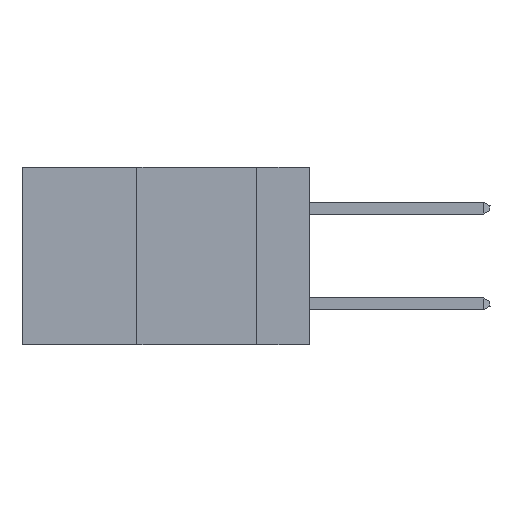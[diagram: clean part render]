
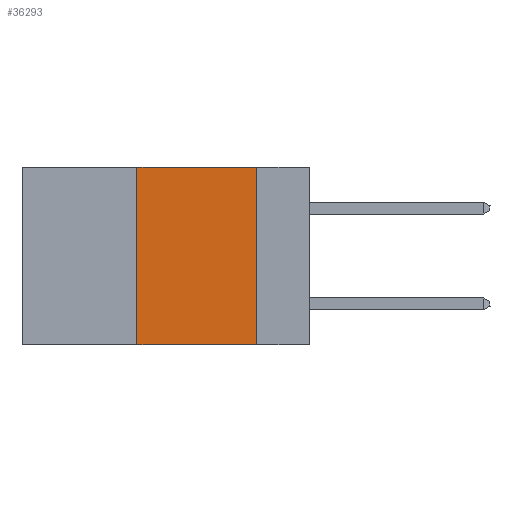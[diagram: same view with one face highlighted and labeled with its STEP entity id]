
A CAD part, left-side view. The second image highlights one B-rep face of the part: STEP entity #36293.
In plain terms, the highlighted planar face has unit normal (-1, 0, 0).
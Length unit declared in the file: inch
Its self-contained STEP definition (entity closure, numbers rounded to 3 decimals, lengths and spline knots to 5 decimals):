
#799 = AXIS2_PLACEMENT_3D ( 'NONE', #21598, #14729, #39041 ) ;
#840 = PLANE ( 'NONE',  #799 ) ;
#2633 = EDGE_CURVE ( 'NONE', #2727, #32750, #8360, .T. ) ;
#2727 = VERTEX_POINT ( 'NONE', #3957 ) ;
#2901 = EDGE_CURVE ( 'NONE', #4560, #41221, #14847, .T. ) ;
#3219 = CARTESIAN_POINT ( 'NONE',  ( 0., 0.11, 0. ) ) ;
#3957 = CARTESIAN_POINT ( 'NONE',  ( 0., 0.11, 0. ) ) ;
#4560 = VERTEX_POINT ( 'NONE', #28279 ) ;
#8142 = CARTESIAN_POINT ( 'NONE',  ( 0., 0.36, 0. ) ) ;
#8360 = LINE ( 'NONE', #3219, #17580 ) ;
#9922 = ORIENTED_EDGE ( 'NONE', *, *, #2633, .F. ) ;
#11179 = FACE_OUTER_BOUND ( 'NONE', #34096, .T. ) ;
#13161 = CARTESIAN_POINT ( 'NONE',  ( 0., 0.11, -0.37 ) ) ;
#13806 = EDGE_CURVE ( 'NONE', #41221, #2727, #28674, .T. ) ;
#14729 = DIRECTION ( 'NONE',  ( 1., 0., 0. ) ) ;
#14847 = LINE ( 'NONE', #8142, #33311 ) ;
#17580 = VECTOR ( 'NONE', #20487, 39.37008 ) ;
#19437 = VECTOR ( 'NONE', #35795, 39.37008 ) ;
#19886 = ORIENTED_EDGE ( 'NONE', *, *, #37817, .T. ) ;
#20173 = CARTESIAN_POINT ( 'NONE',  ( 0., 0.6, -0.37 ) ) ;
#20487 = DIRECTION ( 'NONE',  ( 0., 0., -1. ) ) ;
#21598 = CARTESIAN_POINT ( 'NONE',  ( 0., 0.6, 0. ) ) ;
#21932 = VECTOR ( 'NONE', #44381, 39.37008 ) ;
#21962 = ORIENTED_EDGE ( 'NONE', *, *, #2901, .F. ) ;
#25228 = ORIENTED_EDGE ( 'NONE', *, *, #13806, .F. ) ;
#28279 = CARTESIAN_POINT ( 'NONE',  ( 0., 0.36, -0.37 ) ) ;
#28674 = LINE ( 'NONE', #39155, #19437 ) ;
#30085 = LINE ( 'NONE', #20173, #21932 ) ;
#32397 = DIRECTION ( 'NONE',  ( 0., 0., 1. ) ) ;
#32750 = VERTEX_POINT ( 'NONE', #13161 ) ;
#33311 = VECTOR ( 'NONE', #32397, 39.37008 ) ;
#34096 = EDGE_LOOP ( 'NONE', ( #9922, #25228, #21962, #19886 ) ) ;
#35795 = DIRECTION ( 'NONE',  ( 0., -1., 0. ) ) ;
#36293 = ADVANCED_FACE ( 'NONE', ( #11179 ), #840, .F. ) ;
#37817 = EDGE_CURVE ( 'NONE', #4560, #32750, #30085, .T. ) ;
#39041 = DIRECTION ( 'NONE',  ( 0., 0., -1. ) ) ;
#39155 = CARTESIAN_POINT ( 'NONE',  ( 0., 0.6, 0. ) ) ;
#40063 = CARTESIAN_POINT ( 'NONE',  ( 0., 0.36, 0. ) ) ;
#41221 = VERTEX_POINT ( 'NONE', #40063 ) ;
#44381 = DIRECTION ( 'NONE',  ( 0., -1., 0. ) ) ;
